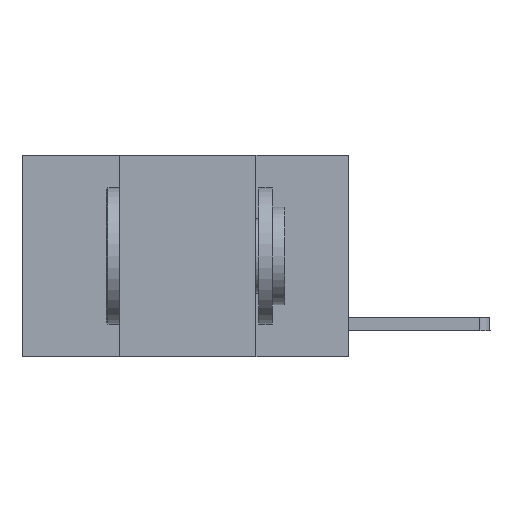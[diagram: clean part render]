
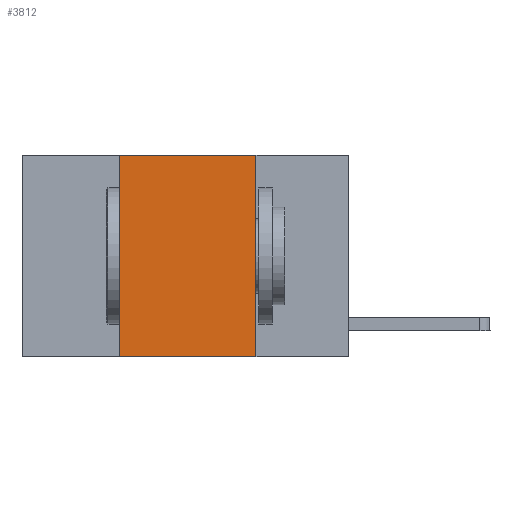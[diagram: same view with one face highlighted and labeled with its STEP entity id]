
A CAD part, left-side view. The second image highlights one B-rep face of the part: STEP entity #3812.
In plain terms, the highlighted planar face has unit normal (-1, 0, 0).
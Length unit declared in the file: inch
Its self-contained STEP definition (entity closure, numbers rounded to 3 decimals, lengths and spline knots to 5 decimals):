
#214 = CARTESIAN_POINT ( 'NONE',  ( 0., 0.42, 0. ) ) ;
#356 = VECTOR ( 'NONE', #6070, 39.37008 ) ;
#553 = VECTOR ( 'NONE', #5003, 39.37008 ) ;
#610 = EDGE_CURVE ( 'NONE', #2312, #3756, #8322, .T. ) ;
#972 = LINE ( 'NONE', #6185, #2796 ) ;
#1282 = DIRECTION ( 'NONE',  ( 0., 0., -1. ) ) ;
#1378 = CARTESIAN_POINT ( 'NONE',  ( 0., 0.17, 0. ) ) ;
#2312 = VERTEX_POINT ( 'NONE', #8276 ) ;
#2610 = EDGE_LOOP ( 'NONE', ( #10395, #8387, #6576, #5417 ) ) ;
#2796 = VECTOR ( 'NONE', #5246, 39.37008 ) ;
#2980 = CARTESIAN_POINT ( 'NONE',  ( 0., 0.6, 0. ) ) ;
#3142 = EDGE_CURVE ( 'NONE', #8372, #3862, #6939, .T. ) ;
#3157 = EDGE_CURVE ( 'NONE', #2312, #3862, #10368, .T. ) ;
#3756 = VERTEX_POINT ( 'NONE', #11022 ) ;
#3812 = ADVANCED_FACE ( 'NONE', ( #3880 ), #5022, .F. ) ;
#3862 = VERTEX_POINT ( 'NONE', #4900 ) ;
#3880 = FACE_OUTER_BOUND ( 'NONE', #2610, .T. ) ;
#4900 = CARTESIAN_POINT ( 'NONE',  ( 0., 0.17, -0.37 ) ) ;
#5003 = DIRECTION ( 'NONE',  ( 0., 0., -1. ) ) ;
#5022 = PLANE ( 'NONE',  #10406 ) ;
#5246 = DIRECTION ( 'NONE',  ( 0., -1., 0. ) ) ;
#5417 = ORIENTED_EDGE ( 'NONE', *, *, #3157, .T. ) ;
#6070 = DIRECTION ( 'NONE',  ( 0., -1., 0. ) ) ;
#6185 = CARTESIAN_POINT ( 'NONE',  ( 0., 0.6, 0. ) ) ;
#6372 = CARTESIAN_POINT ( 'NONE',  ( 0., 0.17, 0. ) ) ;
#6576 = ORIENTED_EDGE ( 'NONE', *, *, #610, .F. ) ;
#6939 = LINE ( 'NONE', #1378, #553 ) ;
#7430 = DIRECTION ( 'NONE',  ( 0., 0., 1. ) ) ;
#8276 = CARTESIAN_POINT ( 'NONE',  ( 0., 0.42, -0.37 ) ) ;
#8322 = LINE ( 'NONE', #214, #11244 ) ;
#8372 = VERTEX_POINT ( 'NONE', #6372 ) ;
#8387 = ORIENTED_EDGE ( 'NONE', *, *, #11119, .F. ) ;
#10368 = LINE ( 'NONE', #10547, #356 ) ;
#10395 = ORIENTED_EDGE ( 'NONE', *, *, #3142, .F. ) ;
#10406 = AXIS2_PLACEMENT_3D ( 'NONE', #2980, #11080, #1282 ) ;
#10547 = CARTESIAN_POINT ( 'NONE',  ( 0., 0.6, -0.37 ) ) ;
#11022 = CARTESIAN_POINT ( 'NONE',  ( 0., 0.42, 0. ) ) ;
#11080 = DIRECTION ( 'NONE',  ( 1., 0., 0. ) ) ;
#11119 = EDGE_CURVE ( 'NONE', #3756, #8372, #972, .T. ) ;
#11244 = VECTOR ( 'NONE', #7430, 39.37008 ) ;
